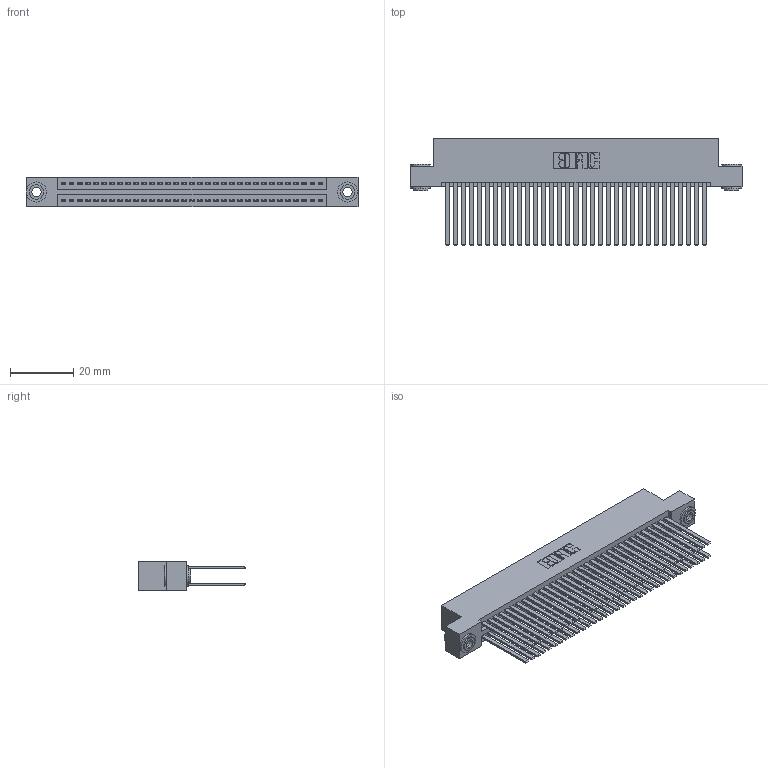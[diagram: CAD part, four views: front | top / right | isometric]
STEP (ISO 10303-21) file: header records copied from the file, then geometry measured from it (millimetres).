
FILE_DESCRIPTION (( 'STEP AP203' ), '1' );
FILE_NAME ('345-066-544-203.STEP', '2019-10-30T17:37:32', ( '' ), ( '' ), 'SwSTEP 2.0', 'SolidWorks 2016', '' );
FILE_SCHEMA (( 'CONFIG_CONTROL_DESIGN' ));
Length unit declared in the file: inch
Products named in the file (4): 345 Part_Flush Mounting Lugs - 0.156 Dia-TH; 345-066-544-203; 345-250-002_345-250-002-102; 345-292-001_345-293-144
Assembly tree (69 placements, depth 2):
  345-066-544-203
    345 Part_Flush Mounting Lugs - 0.156 Dia-TH
    345-292-001_345-293-144  x66
    345-250-002_345-250-002-102  x2
Bounding box: 105.03 x 33.96 x 9.4 mm (x, y, z)
Volume: 11063.7 mm3; surface area: 19096.2 mm2
Topology: 69 solids, 69 shells, 3068 faces, 9063 edges, 5950 vertices
Faces by surface type: plane 2004, cylinder 1056, cone 8
Entity records: 27570 total; most frequent: CARTESIAN_POINT 4603, ORIENTED_EDGE 4530, DIRECTION 4099, EDGE_CURVE 2265, LINE 1981, VECTOR 1981, VERTEX_POINT 1506, AXIS2_PLACEMENT_3D 1059
